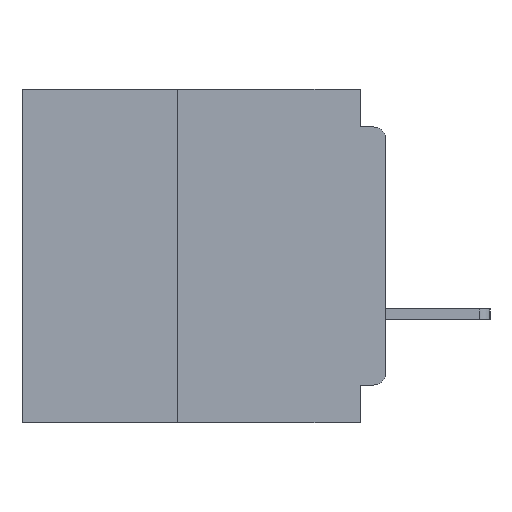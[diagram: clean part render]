
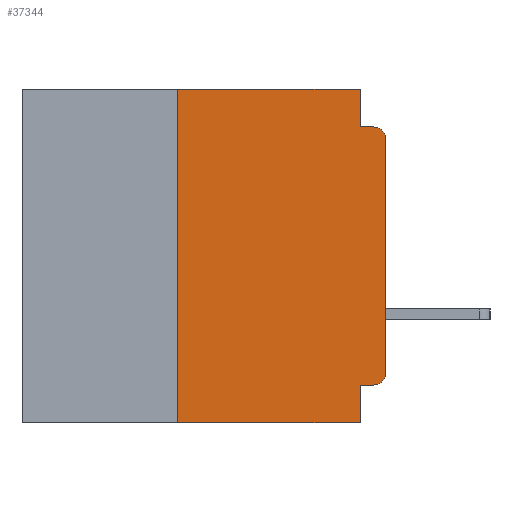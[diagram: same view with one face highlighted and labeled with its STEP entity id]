
A CAD part, left-side view. The second image highlights one B-rep face of the part: STEP entity #37344.
In plain terms, the highlighted planar face has unit normal (-1, 0, 0).
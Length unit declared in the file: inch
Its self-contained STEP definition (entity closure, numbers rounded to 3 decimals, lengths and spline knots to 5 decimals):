
#1139 = LINE ( 'NONE', #39942, #8454 ) ;
#2133 = VERTEX_POINT ( 'NONE', #43754 ) ;
#2527 = VERTEX_POINT ( 'NONE', #34770 ) ;
#2763 = EDGE_LOOP ( 'NONE', ( #42211, #18149, #13206, #41671, #19879, #17092, #39455, #30557, #44510, #11730 ) ) ;
#3525 = EDGE_CURVE ( 'NONE', #38855, #2133, #43605, .T. ) ;
#3737 = AXIS2_PLACEMENT_3D ( 'NONE', #13508, #38448, #17038 ) ;
#5350 = DIRECTION ( 'NONE',  ( 0., -1., 0. ) ) ;
#6235 = DIRECTION ( 'NONE',  ( -1., 0., 0. ) ) ;
#6384 = EDGE_CURVE ( 'NONE', #20743, #45476, #21036, .T. ) ;
#7588 = CARTESIAN_POINT ( 'NONE',  ( 0., 0.031, -0.045 ) ) ;
#7712 = VECTOR ( 'NONE', #17879, 39.37008 ) ;
#7717 = CARTESIAN_POINT ( 'NONE',  ( 0., 0.25, 0. ) ) ;
#8454 = VECTOR ( 'NONE', #25728, 39.37008 ) ;
#8544 = CARTESIAN_POINT ( 'NONE',  ( 0., 0., 0. ) ) ;
#8721 = CARTESIAN_POINT ( 'NONE',  ( 0., 0., -0.045 ) ) ;
#11563 = VECTOR ( 'NONE', #26792, 39.37008 ) ;
#11730 = ORIENTED_EDGE ( 'NONE', *, *, #39106, .T. ) ;
#12126 = DIRECTION ( 'NONE',  ( 0., 0., 1. ) ) ;
#12384 = CARTESIAN_POINT ( 'NONE',  ( 0., 0.437, 0. ) ) ;
#12876 = VERTEX_POINT ( 'NONE', #7588 ) ;
#12933 = VECTOR ( 'NONE', #13246, 39.37008 ) ;
#13140 = CARTESIAN_POINT ( 'NONE',  ( 0., 0., -0.355 ) ) ;
#13206 = ORIENTED_EDGE ( 'NONE', *, *, #24908, .F. ) ;
#13246 = DIRECTION ( 'NONE',  ( 0., 1., 0. ) ) ;
#13508 = CARTESIAN_POINT ( 'NONE',  ( 0., 0.437, 0. ) ) ;
#13527 = VERTEX_POINT ( 'NONE', #41621 ) ;
#13698 = VERTEX_POINT ( 'NONE', #31945 ) ;
#14101 = FACE_OUTER_BOUND ( 'NONE', #2763, .T. ) ;
#15019 = VECTOR ( 'NONE', #5350, 39.37008 ) ;
#15689 = VERTEX_POINT ( 'NONE', #7717 ) ;
#15871 = DIRECTION ( 'NONE',  ( 0., 0., 1. ) ) ;
#15949 = VECTOR ( 'NONE', #12126, 39.37008 ) ;
#17035 = LINE ( 'NONE', #8544, #15949 ) ;
#17038 = DIRECTION ( 'NONE',  ( 0., 0., -1. ) ) ;
#17092 = ORIENTED_EDGE ( 'NONE', *, *, #41226, .F. ) ;
#17417 = EDGE_CURVE ( 'NONE', #2527, #45773, #17035, .T. ) ;
#17835 = CIRCLE ( 'NONE', #32641, 0.015 ) ;
#17879 = DIRECTION ( 'NONE',  ( 0., 0., -1. ) ) ;
#18149 = ORIENTED_EDGE ( 'NONE', *, *, #32352, .T. ) ;
#18170 = DIRECTION ( 'NONE',  ( -1., 0., 0. ) ) ;
#18811 = LINE ( 'NONE', #8721, #42847 ) ;
#19879 = ORIENTED_EDGE ( 'NONE', *, *, #40189, .F. ) ;
#20743 = VERTEX_POINT ( 'NONE', #31666 ) ;
#21036 = LINE ( 'NONE', #27804, #11563 ) ;
#22932 = CIRCLE ( 'NONE', #25614, 0.015 ) ;
#24641 = EDGE_CURVE ( 'NONE', #13698, #12876, #45650, .T. ) ;
#24908 = EDGE_CURVE ( 'NONE', #12876, #13527, #18811, .T. ) ;
#25614 = AXIS2_PLACEMENT_3D ( 'NONE', #27597, #6235, #31207 ) ;
#25728 = DIRECTION ( 'NONE',  ( 0., 0., -1. ) ) ;
#26792 = DIRECTION ( 'NONE',  ( 0., -1., 0. ) ) ;
#27597 = CARTESIAN_POINT ( 'NONE',  ( 0., 0.015, -0.34 ) ) ;
#27675 = PLANE ( 'NONE',  #3737 ) ;
#27804 = CARTESIAN_POINT ( 'NONE',  ( 0., 0.437, -0.4 ) ) ;
#29682 = CARTESIAN_POINT ( 'NONE',  ( 0., 0.015, -0.355 ) ) ;
#30557 = ORIENTED_EDGE ( 'NONE', *, *, #46183, .F. ) ;
#31207 = DIRECTION ( 'NONE',  ( 0., 0., -1. ) ) ;
#31666 = CARTESIAN_POINT ( 'NONE',  ( 0., 0.25, -0.4 ) ) ;
#31945 = CARTESIAN_POINT ( 'NONE',  ( 0., 0.031, 0. ) ) ;
#32352 = EDGE_CURVE ( 'NONE', #45773, #13527, #17835, .T. ) ;
#32641 = AXIS2_PLACEMENT_3D ( 'NONE', #39586, #18170, #43163 ) ;
#33691 = DIRECTION ( 'NONE',  ( 0., -1., 0. ) ) ;
#34007 = VECTOR ( 'NONE', #15871, 39.37008 ) ;
#34770 = CARTESIAN_POINT ( 'NONE',  ( 0., 0., -0.34 ) ) ;
#35204 = CARTESIAN_POINT ( 'NONE',  ( 0., 0.031, -0.4 ) ) ;
#36253 = LINE ( 'NONE', #12384, #15019 ) ;
#37227 = CARTESIAN_POINT ( 'NONE',  ( 0., 0.25, -0.4 ) ) ;
#37344 = ADVANCED_FACE ( 'NONE', ( #14101 ), #27675, .F. ) ;
#38448 = DIRECTION ( 'NONE',  ( 1., 0., 0. ) ) ;
#38855 = VERTEX_POINT ( 'NONE', #29682 ) ;
#39106 = EDGE_CURVE ( 'NONE', #38855, #2527, #22932, .T. ) ;
#39455 = ORIENTED_EDGE ( 'NONE', *, *, #6384, .T. ) ;
#39586 = CARTESIAN_POINT ( 'NONE',  ( 0., 0.015, -0.06 ) ) ;
#39942 = CARTESIAN_POINT ( 'NONE',  ( 0., 0.031, -0.4 ) ) ;
#40189 = EDGE_CURVE ( 'NONE', #15689, #13698, #36253, .T. ) ;
#40444 = CARTESIAN_POINT ( 'NONE',  ( 0., 0., -0.06 ) ) ;
#41226 = EDGE_CURVE ( 'NONE', #20743, #15689, #43454, .T. ) ;
#41621 = CARTESIAN_POINT ( 'NONE',  ( 0., 0.015, -0.045 ) ) ;
#41671 = ORIENTED_EDGE ( 'NONE', *, *, #24641, .F. ) ;
#42211 = ORIENTED_EDGE ( 'NONE', *, *, #17417, .T. ) ;
#42847 = VECTOR ( 'NONE', #33691, 39.37008 ) ;
#43163 = DIRECTION ( 'NONE',  ( 0., 0., -1. ) ) ;
#43454 = LINE ( 'NONE', #37227, #34007 ) ;
#43605 = LINE ( 'NONE', #13140, #12933 ) ;
#43754 = CARTESIAN_POINT ( 'NONE',  ( 0., 0.031, -0.355 ) ) ;
#44510 = ORIENTED_EDGE ( 'NONE', *, *, #3525, .F. ) ;
#45476 = VERTEX_POINT ( 'NONE', #35204 ) ;
#45650 = LINE ( 'NONE', #46294, #7712 ) ;
#45773 = VERTEX_POINT ( 'NONE', #40444 ) ;
#46183 = EDGE_CURVE ( 'NONE', #2133, #45476, #1139, .T. ) ;
#46294 = CARTESIAN_POINT ( 'NONE',  ( 0., 0.031, 0. ) ) ;
